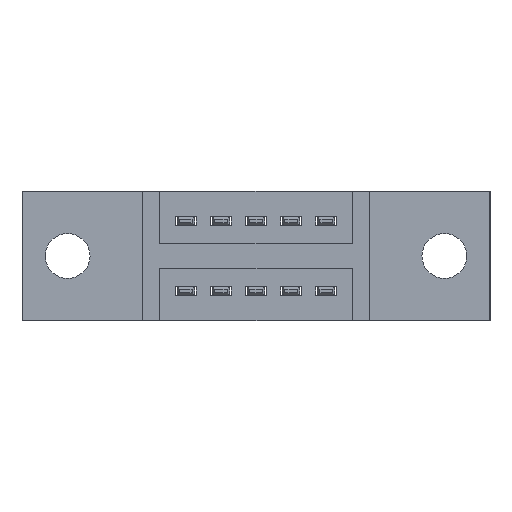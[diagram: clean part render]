
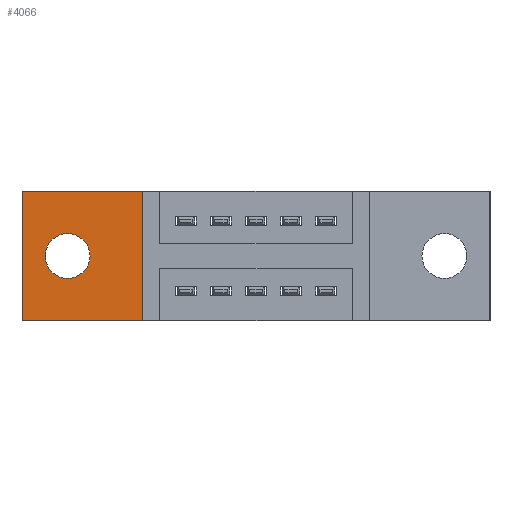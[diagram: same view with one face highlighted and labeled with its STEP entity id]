
A CAD part, front view. The second image highlights one B-rep face of the part: STEP entity #4066.
In plain terms, the highlighted planar face has unit normal (0, -1, 0).
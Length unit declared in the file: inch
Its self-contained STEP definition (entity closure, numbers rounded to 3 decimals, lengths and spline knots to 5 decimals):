
#572 = ORIENTED_EDGE ( 'NONE', *, *, #1843, .F. ) ;
#619 = CARTESIAN_POINT ( 'NONE',  ( 0., 0.11, -0.37 ) ) ;
#666 = VERTEX_POINT ( 'NONE', #2535 ) ;
#689 = VERTEX_POINT ( 'NONE', #2834 ) ;
#923 = VERTEX_POINT ( 'NONE', #1197 ) ;
#1124 = VERTEX_POINT ( 'NONE', #8617 ) ;
#1197 = CARTESIAN_POINT ( 'NONE',  ( 0.3425, 0.11, -0.37 ) ) ;
#1318 = CARTESIAN_POINT ( 'NONE',  ( 0., 0.11, 0. ) ) ;
#1484 = DIRECTION ( 'NONE',  ( -1., 0., 0. ) ) ;
#1501 = CIRCLE ( 'NONE', #4594, 0.064 ) ;
#1843 = EDGE_CURVE ( 'NONE', #689, #1124, #1501, .T. ) ;
#2094 = DIRECTION ( 'NONE',  ( 1., 0., 0. ) ) ;
#2248 = ORIENTED_EDGE ( 'NONE', *, *, #3502, .T. ) ;
#2257 = ORIENTED_EDGE ( 'NONE', *, *, #5246, .F. ) ;
#2535 = CARTESIAN_POINT ( 'NONE',  ( 0., 0.11, 0. ) ) ;
#2554 = VERTEX_POINT ( 'NONE', #5879 ) ;
#2703 = AXIS2_PLACEMENT_3D ( 'NONE', #3516, #5891, #4062 ) ;
#2834 = CARTESIAN_POINT ( 'NONE',  ( 0.13, 0.11, -0.249 ) ) ;
#3212 = DIRECTION ( 'NONE',  ( 0., -1., 0. ) ) ;
#3502 = EDGE_CURVE ( 'NONE', #923, #2554, #8327, .T. ) ;
#3516 = CARTESIAN_POINT ( 'NONE',  ( 0.13, 0.11, -0.185 ) ) ;
#4062 = DIRECTION ( 'NONE',  ( 0., 0., -1. ) ) ;
#4066 = ADVANCED_FACE ( 'NONE', ( #8567, #5281 ), #6076, .T. ) ;
#4081 = VECTOR ( 'NONE', #1484, 39.37008 ) ;
#4162 = CARTESIAN_POINT ( 'NONE',  ( 0., 0.11, -0.37 ) ) ;
#4594 = AXIS2_PLACEMENT_3D ( 'NONE', #7852, #3212, #5979 ) ;
#4795 = AXIS2_PLACEMENT_3D ( 'NONE', #6168, #6187, #5482 ) ;
#5032 = EDGE_CURVE ( 'NONE', #2554, #666, #8050, .T. ) ;
#5246 = EDGE_CURVE ( 'NONE', #1124, #689, #7725, .T. ) ;
#5281 = FACE_OUTER_BOUND ( 'NONE', #8358, .T. ) ;
#5482 = DIRECTION ( 'NONE',  ( 0., 0., -1. ) ) ;
#5650 = CARTESIAN_POINT ( 'NONE',  ( 0.3425, 0.11, 0. ) ) ;
#5680 = LINE ( 'NONE', #1318, #7605 ) ;
#5879 = CARTESIAN_POINT ( 'NONE',  ( 0.3425, 0.11, 0. ) ) ;
#5891 = DIRECTION ( 'NONE',  ( 0., -1., 0. ) ) ;
#5979 = DIRECTION ( 'NONE',  ( 0., 0., -1. ) ) ;
#6076 = PLANE ( 'NONE',  #4795 ) ;
#6168 = CARTESIAN_POINT ( 'NONE',  ( 0., 0.11, -0.37 ) ) ;
#6187 = DIRECTION ( 'NONE',  ( 0., -1., 0. ) ) ;
#6389 = EDGE_CURVE ( 'NONE', #666, #7022, #5680, .T. ) ;
#6998 = EDGE_CURVE ( 'NONE', #7022, #923, #7494, .T. ) ;
#7022 = VERTEX_POINT ( 'NONE', #4162 ) ;
#7338 = ORIENTED_EDGE ( 'NONE', *, *, #6389, .T. ) ;
#7494 = LINE ( 'NONE', #619, #8290 ) ;
#7605 = VECTOR ( 'NONE', #8070, 39.37008 ) ;
#7653 = ORIENTED_EDGE ( 'NONE', *, *, #6998, .T. ) ;
#7725 = CIRCLE ( 'NONE', #2703, 0.064 ) ;
#7729 = ORIENTED_EDGE ( 'NONE', *, *, #5032, .T. ) ;
#7852 = CARTESIAN_POINT ( 'NONE',  ( 0.13, 0.11, -0.185 ) ) ;
#8043 = DIRECTION ( 'NONE',  ( 0., 0., 1. ) ) ;
#8050 = LINE ( 'NONE', #8357, #4081 ) ;
#8070 = DIRECTION ( 'NONE',  ( 0., 0., -1. ) ) ;
#8125 = VECTOR ( 'NONE', #8043, 39.37008 ) ;
#8290 = VECTOR ( 'NONE', #2094, 39.37008 ) ;
#8327 = LINE ( 'NONE', #5650, #8125 ) ;
#8357 = CARTESIAN_POINT ( 'NONE',  ( 0., 0.11, 0. ) ) ;
#8358 = EDGE_LOOP ( 'NONE', ( #7338, #7653, #2248, #7729 ) ) ;
#8567 = FACE_BOUND ( 'NONE', #8789, .T. ) ;
#8617 = CARTESIAN_POINT ( 'NONE',  ( 0.13, 0.11, -0.121 ) ) ;
#8789 = EDGE_LOOP ( 'NONE', ( #2257, #572 ) ) ;
